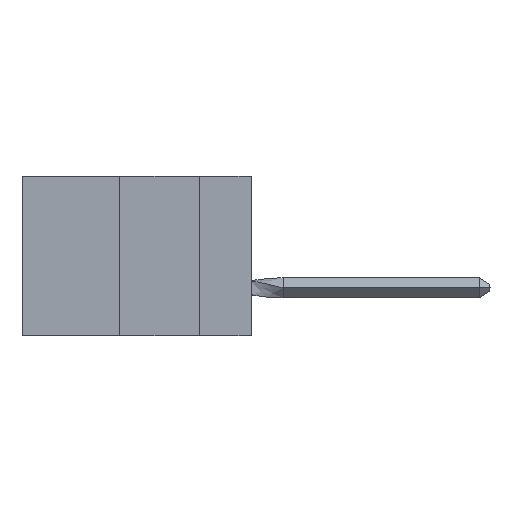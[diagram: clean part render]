
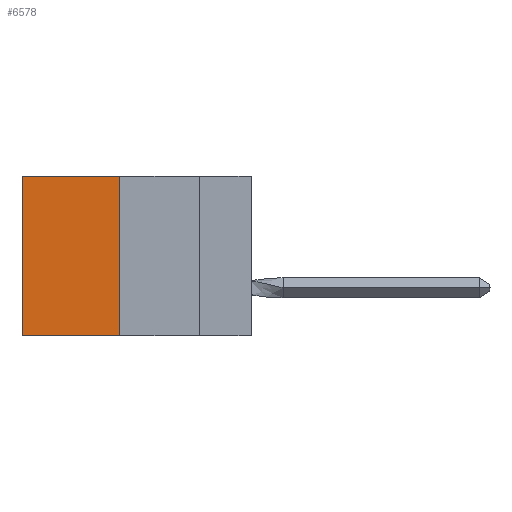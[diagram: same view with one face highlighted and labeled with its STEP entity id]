
A CAD part, left-side view. The second image highlights one B-rep face of the part: STEP entity #6578.
In plain terms, the highlighted planar face has unit normal (-1, 0, 0).
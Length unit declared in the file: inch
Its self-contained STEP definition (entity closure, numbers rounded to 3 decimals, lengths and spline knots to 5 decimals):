
#795 = ORIENTED_EDGE ( 'NONE', *, *, #15899, .T. ) ;
#1063 = LINE ( 'NONE', #11509, #2518 ) ;
#1270 = ORIENTED_EDGE ( 'NONE', *, *, #11592, .F. ) ;
#1535 = ORIENTED_EDGE ( 'NONE', *, *, #17297, .T. ) ;
#1630 = DIRECTION ( 'NONE',  ( 0., 0., -1. ) ) ;
#2011 = CARTESIAN_POINT ( 'NONE',  ( 0.305, 0.413, -0.5 ) ) ;
#2206 = VERTEX_POINT ( 'NONE', #12275 ) ;
#2518 = VECTOR ( 'NONE', #16830, 39.37008 ) ;
#3471 = ORIENTED_EDGE ( 'NONE', *, *, #15773, .F. ) ;
#3581 = VERTEX_POINT ( 'NONE', #3967 ) ;
#3687 = CARTESIAN_POINT ( 'NONE',  ( 0.305, 0.413, -0.5 ) ) ;
#3708 = CARTESIAN_POINT ( 'NONE',  ( 0.305, 0.72, -0.5 ) ) ;
#3967 = CARTESIAN_POINT ( 'NONE',  ( 0.305, 0.413, -0.5 ) ) ;
#4157 = FACE_OUTER_BOUND ( 'NONE', #12221, .T. ) ;
#4486 = VECTOR ( 'NONE', #11731, 39.37008 ) ;
#6429 = DIRECTION ( 'NONE',  ( 0., 0., -1. ) ) ;
#6578 = ADVANCED_FACE ( 'NONE', ( #4157 ), #14672, .F. ) ;
#6768 = VECTOR ( 'NONE', #1630, 39.37008 ) ;
#7659 = VECTOR ( 'NONE', #11498, 39.37008 ) ;
#8083 = LINE ( 'NONE', #9045, #4486 ) ;
#8415 = CARTESIAN_POINT ( 'NONE',  ( 0.305, 0.72, -0.5 ) ) ;
#9045 = CARTESIAN_POINT ( 'NONE',  ( 0.305, 0.413, 0. ) ) ;
#9255 = DIRECTION ( 'NONE',  ( 1., 0., 0. ) ) ;
#11498 = DIRECTION ( 'NONE',  ( 0., 0., -1. ) ) ;
#11509 = CARTESIAN_POINT ( 'NONE',  ( 0.305, 0.413, -0.5 ) ) ;
#11592 = EDGE_CURVE ( 'NONE', #3581, #13670, #1063, .T. ) ;
#11631 = VERTEX_POINT ( 'NONE', #12972 ) ;
#11731 = DIRECTION ( 'NONE',  ( 0., 1., 0. ) ) ;
#12221 = EDGE_LOOP ( 'NONE', ( #1535, #1270, #3471, #795 ) ) ;
#12275 = CARTESIAN_POINT ( 'NONE',  ( 0.305, 0.72, 0. ) ) ;
#12971 = LINE ( 'NONE', #2011, #7659 ) ;
#12972 = CARTESIAN_POINT ( 'NONE',  ( 0.305, 0.413, 0. ) ) ;
#13670 = VERTEX_POINT ( 'NONE', #3708 ) ;
#14128 = AXIS2_PLACEMENT_3D ( 'NONE', #3687, #9255, #6429 ) ;
#14672 = PLANE ( 'NONE',  #14128 ) ;
#15677 = LINE ( 'NONE', #8415, #6768 ) ;
#15773 = EDGE_CURVE ( 'NONE', #11631, #3581, #12971, .T. ) ;
#15899 = EDGE_CURVE ( 'NONE', #11631, #2206, #8083, .T. ) ;
#16830 = DIRECTION ( 'NONE',  ( 0., 1., 0. ) ) ;
#17297 = EDGE_CURVE ( 'NONE', #2206, #13670, #15677, .T. ) ;
